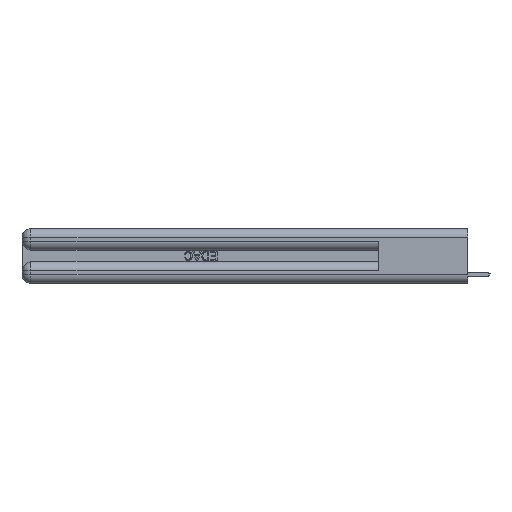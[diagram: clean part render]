
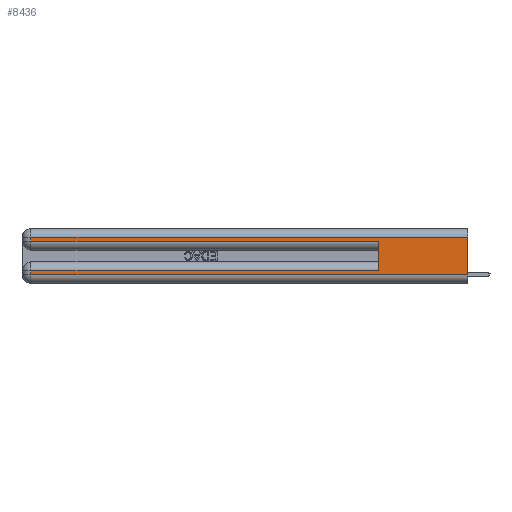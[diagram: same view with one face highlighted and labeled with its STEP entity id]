
A CAD part, left-side view. The second image highlights one B-rep face of the part: STEP entity #8436.
In plain terms, the highlighted planar face has unit normal (-1, 0, 0).
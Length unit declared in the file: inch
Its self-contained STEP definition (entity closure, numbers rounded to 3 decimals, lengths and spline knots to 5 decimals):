
#1670 = CARTESIAN_POINT ( 'NONE',  ( 0., 0., 0.06 ) ) ;
#2486 = CARTESIAN_POINT ( 'NONE',  ( 0., 2.94, 0.285 ) ) ;
#2821 = VERTEX_POINT ( 'NONE', #14818 ) ;
#3021 = LINE ( 'NONE', #31828, #32334 ) ;
#4195 = AXIS2_PLACEMENT_3D ( 'NONE', #33733, #20741, #23096 ) ;
#4218 = EDGE_CURVE ( 'NONE', #22326, #23893, #24135, .T. ) ;
#4225 = CARTESIAN_POINT ( 'NONE',  ( 0., 0., 0.31 ) ) ;
#4371 = EDGE_LOOP ( 'NONE', ( #7976, #27403, #15190, #18893, #8265, #22983, #12434, #6887 ) ) ;
#5284 = LINE ( 'NONE', #32649, #9901 ) ;
#5622 = DIRECTION ( 'NONE',  ( 0., 0., 1. ) ) ;
#6887 = ORIENTED_EDGE ( 'NONE', *, *, #8549, .T. ) ;
#6942 = VECTOR ( 'NONE', #5622, 39.37008 ) ;
#7843 = CARTESIAN_POINT ( 'NONE',  ( 0., 0., 0.085 ) ) ;
#7976 = ORIENTED_EDGE ( 'NONE', *, *, #27844, .F. ) ;
#8033 = CARTESIAN_POINT ( 'NONE',  ( 0., 2.94, 0.085 ) ) ;
#8265 = ORIENTED_EDGE ( 'NONE', *, *, #26907, .F. ) ;
#8343 = CARTESIAN_POINT ( 'NONE',  ( 0., 2.94, 0.37 ) ) ;
#8436 = ADVANCED_FACE ( 'NONE', ( #10998 ), #20511, .F. ) ;
#8549 = EDGE_CURVE ( 'NONE', #21386, #26817, #3021, .T. ) ;
#9901 = VECTOR ( 'NONE', #27410, 39.37008 ) ;
#10395 = EDGE_CURVE ( 'NONE', #23893, #2821, #16305, .T. ) ;
#10515 = EDGE_CURVE ( 'NONE', #13182, #21386, #26356, .T. ) ;
#10998 = FACE_OUTER_BOUND ( 'NONE', #4371, .T. ) ;
#11539 = CARTESIAN_POINT ( 'NONE',  ( 0., 0., 0.285 ) ) ;
#12081 = CARTESIAN_POINT ( 'NONE',  ( 0., 2.94, 0.37 ) ) ;
#12434 = ORIENTED_EDGE ( 'NONE', *, *, #10515, .T. ) ;
#12987 = DIRECTION ( 'NONE',  ( 0., -1., 0. ) ) ;
#13182 = VERTEX_POINT ( 'NONE', #8033 ) ;
#14818 = CARTESIAN_POINT ( 'NONE',  ( 0., 0.6, 0.285 ) ) ;
#15190 = ORIENTED_EDGE ( 'NONE', *, *, #4218, .T. ) ;
#15310 = CARTESIAN_POINT ( 'NONE',  ( 0., 0., 0.37 ) ) ;
#15879 = VECTOR ( 'NONE', #29882, 39.37008 ) ;
#16246 = VERTEX_POINT ( 'NONE', #4225 ) ;
#16305 = LINE ( 'NONE', #11539, #17984 ) ;
#16392 = CARTESIAN_POINT ( 'NONE',  ( 0., 0.6, 0.145 ) ) ;
#16658 = EDGE_CURVE ( 'NONE', #18898, #13182, #21496, .T. ) ;
#17868 = CARTESIAN_POINT ( 'NONE',  ( 0., 2.94, 0.31 ) ) ;
#17872 = DIRECTION ( 'NONE',  ( 0., 0., -1. ) ) ;
#17984 = VECTOR ( 'NONE', #29966, 39.37008 ) ;
#18604 = LINE ( 'NONE', #15310, #26569 ) ;
#18893 = ORIENTED_EDGE ( 'NONE', *, *, #10395, .T. ) ;
#18898 = VERTEX_POINT ( 'NONE', #29690 ) ;
#19198 = DIRECTION ( 'NONE',  ( 0., 0., -1. ) ) ;
#20511 = PLANE ( 'NONE',  #4195 ) ;
#20741 = DIRECTION ( 'NONE',  ( 1., 0., 0. ) ) ;
#21386 = VERTEX_POINT ( 'NONE', #30977 ) ;
#21496 = LINE ( 'NONE', #7843, #25305 ) ;
#22326 = VERTEX_POINT ( 'NONE', #17868 ) ;
#22983 = ORIENTED_EDGE ( 'NONE', *, *, #16658, .T. ) ;
#23096 = DIRECTION ( 'NONE',  ( 0., 0., -1. ) ) ;
#23893 = VERTEX_POINT ( 'NONE', #2486 ) ;
#24135 = LINE ( 'NONE', #12081, #26656 ) ;
#24331 = DIRECTION ( 'NONE',  ( 0., 1., 0. ) ) ;
#25305 = VECTOR ( 'NONE', #24331, 39.37008 ) ;
#26356 = LINE ( 'NONE', #8343, #15879 ) ;
#26569 = VECTOR ( 'NONE', #17872, 39.37008 ) ;
#26656 = VECTOR ( 'NONE', #19198, 39.37008 ) ;
#26817 = VERTEX_POINT ( 'NONE', #1670 ) ;
#26907 = EDGE_CURVE ( 'NONE', #18898, #2821, #34155, .T. ) ;
#27403 = ORIENTED_EDGE ( 'NONE', *, *, #32014, .T. ) ;
#27410 = DIRECTION ( 'NONE',  ( 0., 1., 0. ) ) ;
#27844 = EDGE_CURVE ( 'NONE', #16246, #26817, #18604, .T. ) ;
#29690 = CARTESIAN_POINT ( 'NONE',  ( 0., 0.6, 0.085 ) ) ;
#29882 = DIRECTION ( 'NONE',  ( 0., 0., -1. ) ) ;
#29966 = DIRECTION ( 'NONE',  ( 0., -1., 0. ) ) ;
#30977 = CARTESIAN_POINT ( 'NONE',  ( 0., 2.94, 0.06 ) ) ;
#31828 = CARTESIAN_POINT ( 'NONE',  ( 0., 0., 0.06 ) ) ;
#32014 = EDGE_CURVE ( 'NONE', #16246, #22326, #5284, .T. ) ;
#32334 = VECTOR ( 'NONE', #12987, 39.37008 ) ;
#32649 = CARTESIAN_POINT ( 'NONE',  ( 0., 0., 0.31 ) ) ;
#33733 = CARTESIAN_POINT ( 'NONE',  ( 0., 0., 0.37 ) ) ;
#34155 = LINE ( 'NONE', #16392, #6942 ) ;
